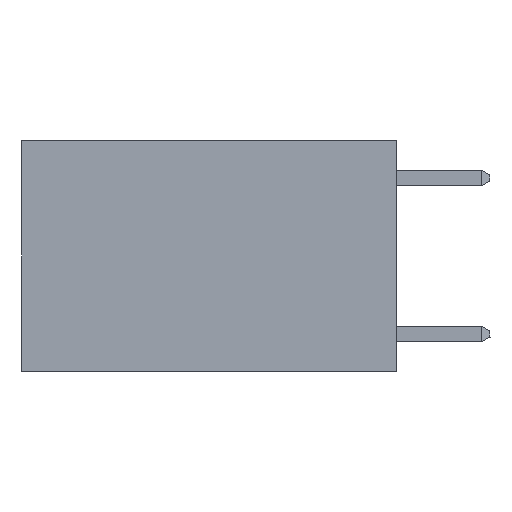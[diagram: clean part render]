
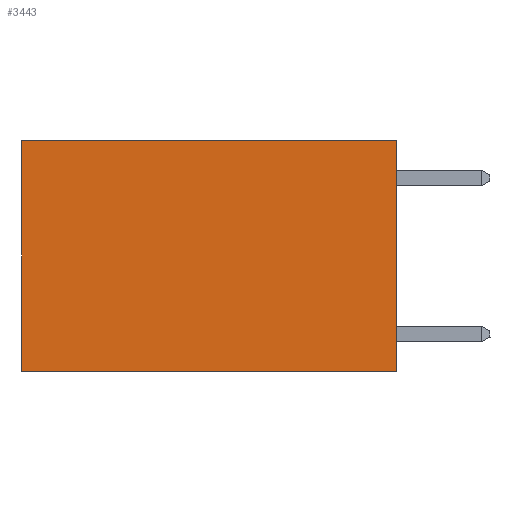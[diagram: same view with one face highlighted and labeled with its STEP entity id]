
A CAD part, left-side view. The second image highlights one B-rep face of the part: STEP entity #3443.
In plain terms, the highlighted planar face has unit normal (-1, 0, 0).
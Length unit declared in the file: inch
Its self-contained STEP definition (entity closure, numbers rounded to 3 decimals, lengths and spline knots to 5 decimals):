
#17 = ORIENTED_EDGE ( 'NONE', *, *, #1993, .T. ) ;
#67 = LINE ( 'NONE', #3740, #9303 ) ;
#95 = EDGE_CURVE ( 'NONE', #2936, #6587, #7925, .T. ) ;
#533 = DIRECTION ( 'NONE',  ( 0., 0., -1. ) ) ;
#617 = DIRECTION ( 'NONE',  ( 1., 0., 0. ) ) ;
#676 = CARTESIAN_POINT ( 'NONE',  ( 0.2625, 0., 0. ) ) ;
#877 = LINE ( 'NONE', #1235, #7800 ) ;
#1050 = LINE ( 'NONE', #3980, #5581 ) ;
#1235 = CARTESIAN_POINT ( 'NONE',  ( 0.2625, 0., 0. ) ) ;
#1503 = VERTEX_POINT ( 'NONE', #4964 ) ;
#1604 = VERTEX_POINT ( 'NONE', #3182 ) ;
#1847 = PLANE ( 'NONE',  #8643 ) ;
#1993 = EDGE_CURVE ( 'NONE', #1503, #6587, #67, .T. ) ;
#2164 = DIRECTION ( 'NONE',  ( 0., 1., 0. ) ) ;
#2936 = VERTEX_POINT ( 'NONE', #7892 ) ;
#3182 = CARTESIAN_POINT ( 'NONE',  ( 0.2625, 0., 0. ) ) ;
#3443 = ADVANCED_FACE ( 'NONE', ( #6454 ), #1847, .F. ) ;
#3740 = CARTESIAN_POINT ( 'NONE',  ( 0.2625, 0.6, 0. ) ) ;
#3749 = ORIENTED_EDGE ( 'NONE', *, *, #95, .F. ) ;
#3940 = DIRECTION ( 'NONE',  ( 0., 0., -1. ) ) ;
#3980 = CARTESIAN_POINT ( 'NONE',  ( 0.2625, 0., 0. ) ) ;
#4235 = DIRECTION ( 'NONE',  ( 0., 1., 0. ) ) ;
#4479 = EDGE_CURVE ( 'NONE', #1604, #2936, #1050, .T. ) ;
#4964 = CARTESIAN_POINT ( 'NONE',  ( 0.2625, 0.6, 0. ) ) ;
#5546 = VECTOR ( 'NONE', #4235, 39.37008 ) ;
#5581 = VECTOR ( 'NONE', #3940, 39.37008 ) ;
#5672 = EDGE_CURVE ( 'NONE', #1604, #1503, #877, .T. ) ;
#6132 = EDGE_LOOP ( 'NONE', ( #17, #3749, #8072, #6502 ) ) ;
#6454 = FACE_OUTER_BOUND ( 'NONE', #6132, .T. ) ;
#6502 = ORIENTED_EDGE ( 'NONE', *, *, #5672, .T. ) ;
#6587 = VERTEX_POINT ( 'NONE', #10376 ) ;
#7800 = VECTOR ( 'NONE', #2164, 39.37008 ) ;
#7892 = CARTESIAN_POINT ( 'NONE',  ( 0.2625, 0., -0.37 ) ) ;
#7925 = LINE ( 'NONE', #8918, #5546 ) ;
#8072 = ORIENTED_EDGE ( 'NONE', *, *, #4479, .F. ) ;
#8643 = AXIS2_PLACEMENT_3D ( 'NONE', #676, #617, #533 ) ;
#8918 = CARTESIAN_POINT ( 'NONE',  ( 0.2625, 0., -0.37 ) ) ;
#9303 = VECTOR ( 'NONE', #11184, 39.37008 ) ;
#10376 = CARTESIAN_POINT ( 'NONE',  ( 0.2625, 0.6, -0.37 ) ) ;
#11184 = DIRECTION ( 'NONE',  ( 0., 0., -1. ) ) ;
